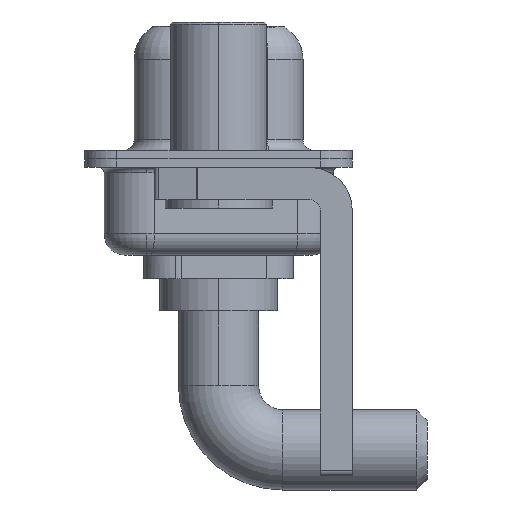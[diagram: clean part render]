
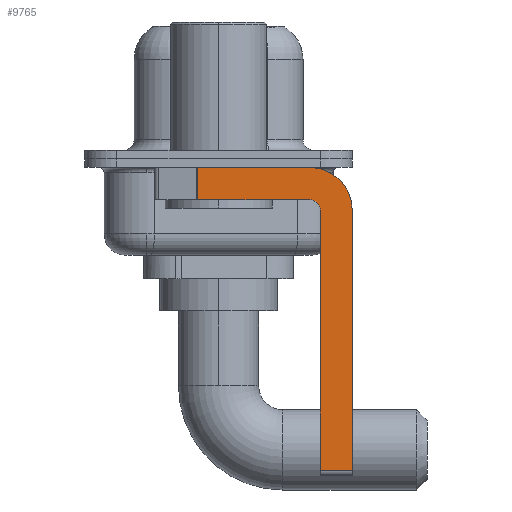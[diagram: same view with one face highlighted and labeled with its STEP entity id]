
A CAD part, left-side view. The second image highlights one B-rep face of the part: STEP entity #9765.
In plain terms, the highlighted planar face has unit normal (-1, 0, 0).
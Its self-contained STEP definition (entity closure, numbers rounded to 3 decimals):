
#522 = VERTEX_POINT ( 'NONE', #4264 ) ;
#626 = ORIENTED_EDGE ( 'NONE', *, *, #13377, .F. ) ;
#645 = EDGE_CURVE ( 'NONE', #13948, #522, #9427, .T. ) ;
#676 = CARTESIAN_POINT ( 'NONE',  ( -2.9, -4.25, -14.55 ) ) ;
#678 = LINE ( 'NONE', #6563, #2059 ) ;
#701 = CARTESIAN_POINT ( 'NONE',  ( -2.9, -4.25, -0.4 ) ) ;
#992 = CARTESIAN_POINT ( 'NONE',  ( -2.9, -4.75, -14.8 ) ) ;
#1680 = VECTOR ( 'NONE', #3115, 1000. ) ;
#1810 = ORIENTED_EDGE ( 'NONE', *, *, #5315, .F. ) ;
#1897 = EDGE_CURVE ( 'NONE', #9089, #13948, #11149, .T. ) ;
#1962 = ORIENTED_EDGE ( 'NONE', *, *, #12985, .F. ) ;
#2004 = DIRECTION ( 'NONE',  ( 0., 1., 0. ) ) ;
#2059 = VECTOR ( 'NONE', #11144, 1000. ) ;
#2126 = LINE ( 'NONE', #9106, #3794 ) ;
#2147 = ORIENTED_EDGE ( 'NONE', *, *, #1897, .F. ) ;
#2452 = DIRECTION ( 'NONE',  ( 0., 0., 1. ) ) ;
#3115 = DIRECTION ( 'NONE',  ( 0., -1., 0. ) ) ;
#3149 = CARTESIAN_POINT ( 'NONE',  ( -2.9, -4.25, -1.9 ) ) ;
#3162 = AXIS2_PLACEMENT_3D ( 'NONE', #11740, #4924, #9482 ) ;
#3794 = VECTOR ( 'NONE', #12557, 1000. ) ;
#3857 = AXIS2_PLACEMENT_3D ( 'NONE', #8882, #14741, #8038 ) ;
#3905 = VECTOR ( 'NONE', #13120, 1000. ) ;
#4264 = CARTESIAN_POINT ( 'NONE',  ( -2.9, -4.25, -1.9 ) ) ;
#4616 = PLANE ( 'NONE',  #3857 ) ;
#4841 = CARTESIAN_POINT ( 'NONE',  ( -2.9, 0.978, -0.4 ) ) ;
#4876 = CARTESIAN_POINT ( 'NONE',  ( -2.9, 0.978, -1.9 ) ) ;
#4924 = DIRECTION ( 'NONE',  ( 1., 0., 0. ) ) ;
#5315 = EDGE_CURVE ( 'NONE', #9012, #12562, #678, .T. ) ;
#5666 = FACE_OUTER_BOUND ( 'NONE', #11314, .T. ) ;
#5898 = CARTESIAN_POINT ( 'NONE',  ( -2.9, -4.75, -2.4 ) ) ;
#6313 = AXIS2_PLACEMENT_3D ( 'NONE', #12736, #6958, #2452 ) ;
#6563 = CARTESIAN_POINT ( 'NONE',  ( -2.9, 3., -0.4 ) ) ;
#6958 = DIRECTION ( 'NONE',  ( -1., 0., 0. ) ) ;
#7059 = VECTOR ( 'NONE', #9937, 1000. ) ;
#7760 = ORIENTED_EDGE ( 'NONE', *, *, #10739, .F. ) ;
#8038 = DIRECTION ( 'NONE',  ( 0., 0., -1. ) ) ;
#8322 = CARTESIAN_POINT ( 'NONE',  ( -2.9, -6.25, -2.4 ) ) ;
#8882 = CARTESIAN_POINT ( 'NONE',  ( -2.9, -4.25, -2.4 ) ) ;
#9012 = VERTEX_POINT ( 'NONE', #4841 ) ;
#9061 = LINE ( 'NONE', #3149, #11249 ) ;
#9089 = VERTEX_POINT ( 'NONE', #11723 ) ;
#9106 = CARTESIAN_POINT ( 'NONE',  ( -2.9, -6.25, -2.4 ) ) ;
#9199 = ORIENTED_EDGE ( 'NONE', *, *, #9589, .T. ) ;
#9427 = CIRCLE ( 'NONE', #6313, 0.5 ) ;
#9448 = ORIENTED_EDGE ( 'NONE', *, *, #12276, .T. ) ;
#9482 = DIRECTION ( 'NONE',  ( 0., 0., -1. ) ) ;
#9589 = EDGE_CURVE ( 'NONE', #9089, #14816, #13389, .T. ) ;
#9765 = ADVANCED_FACE ( 'NONE', ( #5666 ), #4616, .F. ) ;
#9937 = DIRECTION ( 'NONE',  ( 0., 0., 1. ) ) ;
#10042 = CARTESIAN_POINT ( 'NONE',  ( -2.9, -6.25, -14.55 ) ) ;
#10739 = EDGE_CURVE ( 'NONE', #12562, #11898, #11772, .T. ) ;
#11009 = VERTEX_POINT ( 'NONE', #4876 ) ;
#11144 = DIRECTION ( 'NONE',  ( 0., -1., 0. ) ) ;
#11149 = LINE ( 'NONE', #992, #7059 ) ;
#11249 = VECTOR ( 'NONE', #2004, 1000. ) ;
#11314 = EDGE_LOOP ( 'NONE', ( #1810, #9448, #626, #11456, #2147, #9199, #1962, #7760 ) ) ;
#11456 = ORIENTED_EDGE ( 'NONE', *, *, #645, .F. ) ;
#11723 = CARTESIAN_POINT ( 'NONE',  ( -2.9, -4.75, -14.55 ) ) ;
#11740 = CARTESIAN_POINT ( 'NONE',  ( -2.9, -4.25, -2.4 ) ) ;
#11772 = CIRCLE ( 'NONE', #3162, 2. ) ;
#11836 = LINE ( 'NONE', #13951, #3905 ) ;
#11898 = VERTEX_POINT ( 'NONE', #8322 ) ;
#12276 = EDGE_CURVE ( 'NONE', #9012, #11009, #11836, .T. ) ;
#12557 = DIRECTION ( 'NONE',  ( 0., 0., -1. ) ) ;
#12562 = VERTEX_POINT ( 'NONE', #701 ) ;
#12736 = CARTESIAN_POINT ( 'NONE',  ( -2.9, -4.25, -2.4 ) ) ;
#12985 = EDGE_CURVE ( 'NONE', #11898, #14816, #2126, .T. ) ;
#13120 = DIRECTION ( 'NONE',  ( 0., 0., -1. ) ) ;
#13377 = EDGE_CURVE ( 'NONE', #522, #11009, #9061, .T. ) ;
#13389 = LINE ( 'NONE', #676, #1680 ) ;
#13948 = VERTEX_POINT ( 'NONE', #5898 ) ;
#13951 = CARTESIAN_POINT ( 'NONE',  ( -2.9, 0.978, -1.9 ) ) ;
#14741 = DIRECTION ( 'NONE',  ( 1., 0., 0. ) ) ;
#14816 = VERTEX_POINT ( 'NONE', #10042 ) ;
